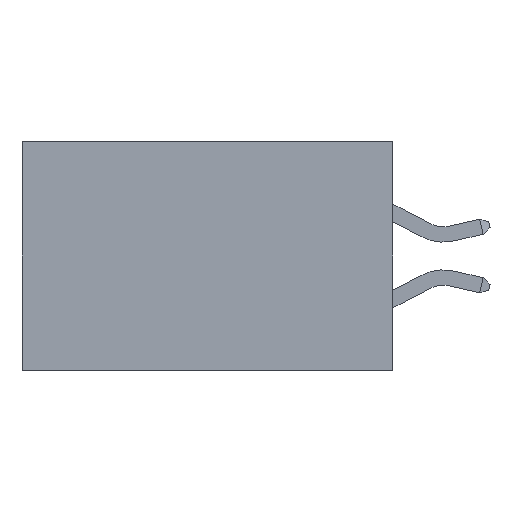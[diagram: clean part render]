
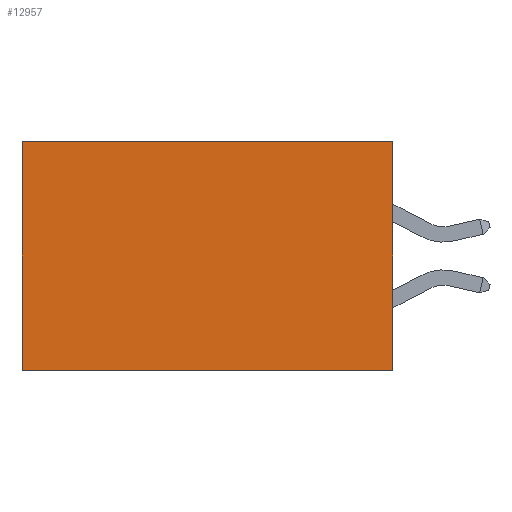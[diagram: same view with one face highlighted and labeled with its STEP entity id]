
A CAD part, left-side view. The second image highlights one B-rep face of the part: STEP entity #12957.
In plain terms, the highlighted planar face has unit normal (-1, 0, 0).
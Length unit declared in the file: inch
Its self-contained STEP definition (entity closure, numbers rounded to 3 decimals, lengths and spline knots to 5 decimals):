
#979 = LINE ( 'NONE', #18790, #32916 ) ;
#1542 = LINE ( 'NONE', #25734, #3622 ) ;
#1949 = LINE ( 'NONE', #29625, #15367 ) ;
#3341 = CARTESIAN_POINT ( 'NONE',  ( 0.2875, 0., 0. ) ) ;
#3622 = VECTOR ( 'NONE', #4010, 39.37008 ) ;
#4010 = DIRECTION ( 'NONE',  ( 0., 0., -1. ) ) ;
#4673 = DIRECTION ( 'NONE',  ( 0., 1., 0. ) ) ;
#5044 = VECTOR ( 'NONE', #4673, 39.37008 ) ;
#6967 = AXIS2_PLACEMENT_3D ( 'NONE', #39354, #26072, #19616 ) ;
#9845 = ORIENTED_EDGE ( 'NONE', *, *, #19483, .F. ) ;
#11125 = VERTEX_POINT ( 'NONE', #36281 ) ;
#11236 = EDGE_LOOP ( 'NONE', ( #26564, #26956, #9845, #15135 ) ) ;
#12957 = ADVANCED_FACE ( 'NONE', ( #37537 ), #32859, .F. ) ;
#15135 = ORIENTED_EDGE ( 'NONE', *, *, #26976, .T. ) ;
#15367 = VECTOR ( 'NONE', #39880, 39.37008 ) ;
#18790 = CARTESIAN_POINT ( 'NONE',  ( 0.2875, 0., 0. ) ) ;
#18928 = LINE ( 'NONE', #39791, #5044 ) ;
#18966 = VERTEX_POINT ( 'NONE', #3341 ) ;
#19142 = CARTESIAN_POINT ( 'NONE',  ( 0.2875, 0.6, -0.37 ) ) ;
#19483 = EDGE_CURVE ( 'NONE', #18966, #11125, #1949, .T. ) ;
#19616 = DIRECTION ( 'NONE',  ( 0., 0., -1. ) ) ;
#22686 = VERTEX_POINT ( 'NONE', #24152 ) ;
#24009 = EDGE_CURVE ( 'NONE', #22686, #39844, #1542, .T. ) ;
#24152 = CARTESIAN_POINT ( 'NONE',  ( 0.2875, 0.6, 0. ) ) ;
#25734 = CARTESIAN_POINT ( 'NONE',  ( 0.2875, 0.6, 0. ) ) ;
#26072 = DIRECTION ( 'NONE',  ( 1., 0., 0. ) ) ;
#26564 = ORIENTED_EDGE ( 'NONE', *, *, #24009, .T. ) ;
#26956 = ORIENTED_EDGE ( 'NONE', *, *, #33102, .F. ) ;
#26976 = EDGE_CURVE ( 'NONE', #18966, #22686, #979, .T. ) ;
#28692 = DIRECTION ( 'NONE',  ( 0., 1., 0. ) ) ;
#29625 = CARTESIAN_POINT ( 'NONE',  ( 0.2875, 0., 0. ) ) ;
#32859 = PLANE ( 'NONE',  #6967 ) ;
#32916 = VECTOR ( 'NONE', #28692, 39.37008 ) ;
#33102 = EDGE_CURVE ( 'NONE', #11125, #39844, #18928, .T. ) ;
#36281 = CARTESIAN_POINT ( 'NONE',  ( 0.2875, 0., -0.37 ) ) ;
#37537 = FACE_OUTER_BOUND ( 'NONE', #11236, .T. ) ;
#39354 = CARTESIAN_POINT ( 'NONE',  ( 0.2875, 0., 0. ) ) ;
#39791 = CARTESIAN_POINT ( 'NONE',  ( 0.2875, 0., -0.37 ) ) ;
#39844 = VERTEX_POINT ( 'NONE', #19142 ) ;
#39880 = DIRECTION ( 'NONE',  ( 0., 0., -1. ) ) ;
